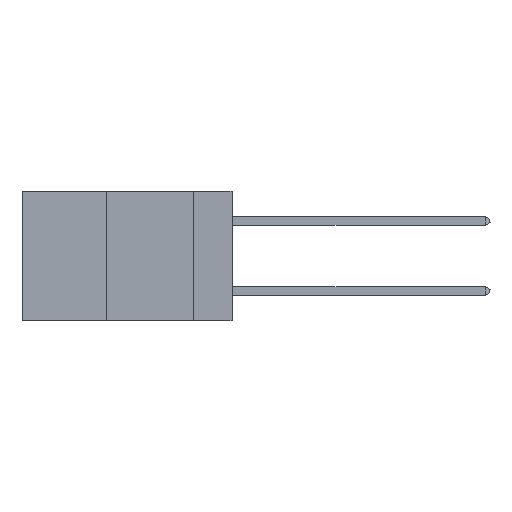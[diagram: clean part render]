
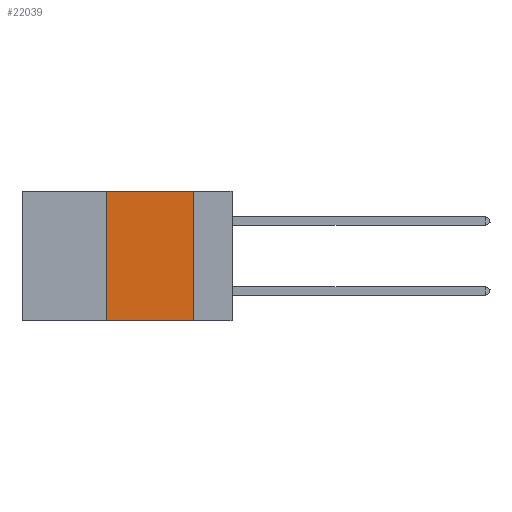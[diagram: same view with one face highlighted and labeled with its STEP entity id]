
A CAD part, left-side view. The second image highlights one B-rep face of the part: STEP entity #22039.
In plain terms, the highlighted planar face has unit normal (-1, 0, 0).
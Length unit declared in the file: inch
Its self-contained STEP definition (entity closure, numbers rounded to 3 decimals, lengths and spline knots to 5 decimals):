
#2424 = CARTESIAN_POINT ( 'NONE',  ( 0., 0.6, -0.37 ) ) ;
#3313 = DIRECTION ( 'NONE',  ( 0., 0., -1. ) ) ;
#3922 = VERTEX_POINT ( 'NONE', #30902 ) ;
#4229 = DIRECTION ( 'NONE',  ( 0., 0., -1. ) ) ;
#4431 = VECTOR ( 'NONE', #3313, 39.37008 ) ;
#4483 = ORIENTED_EDGE ( 'NONE', *, *, #11120, .F. ) ;
#6160 = VECTOR ( 'NONE', #17784, 39.37008 ) ;
#6839 = PLANE ( 'NONE',  #32558 ) ;
#6882 = VECTOR ( 'NONE', #17306, 39.37008 ) ;
#11120 = EDGE_CURVE ( 'NONE', #24749, #3922, #34038, .T. ) ;
#14887 = VECTOR ( 'NONE', #26249, 39.37008 ) ;
#14952 = CARTESIAN_POINT ( 'NONE',  ( 0., 0.6, 0. ) ) ;
#14987 = VERTEX_POINT ( 'NONE', #24565 ) ;
#15161 = CARTESIAN_POINT ( 'NONE',  ( 0., 0.6, 0. ) ) ;
#17306 = DIRECTION ( 'NONE',  ( 0., 0., 1. ) ) ;
#17784 = DIRECTION ( 'NONE',  ( 0., -1., 0. ) ) ;
#17951 = ORIENTED_EDGE ( 'NONE', *, *, #23624, .F. ) ;
#18876 = EDGE_LOOP ( 'NONE', ( #17951, #4483, #28363, #30797 ) ) ;
#19497 = EDGE_CURVE ( 'NONE', #29787, #14987, #21762, .T. ) ;
#20151 = DIRECTION ( 'NONE',  ( 1., 0., 0. ) ) ;
#21762 = LINE ( 'NONE', #2424, #14887 ) ;
#22039 = ADVANCED_FACE ( 'NONE', ( #32158 ), #6839, .F. ) ;
#23624 = EDGE_CURVE ( 'NONE', #3922, #14987, #34014, .T. ) ;
#23632 = CARTESIAN_POINT ( 'NONE',  ( 0., 0.36, 0. ) ) ;
#24507 = CARTESIAN_POINT ( 'NONE',  ( 0., 0.11, 0. ) ) ;
#24565 = CARTESIAN_POINT ( 'NONE',  ( 0., 0.11, -0.37 ) ) ;
#24749 = VERTEX_POINT ( 'NONE', #23632 ) ;
#24965 = CARTESIAN_POINT ( 'NONE',  ( 0., 0.36, 0. ) ) ;
#26249 = DIRECTION ( 'NONE',  ( 0., -1., 0. ) ) ;
#27833 = LINE ( 'NONE', #24965, #6882 ) ;
#28363 = ORIENTED_EDGE ( 'NONE', *, *, #29269, .F. ) ;
#29269 = EDGE_CURVE ( 'NONE', #29787, #24749, #27833, .T. ) ;
#29787 = VERTEX_POINT ( 'NONE', #31382 ) ;
#30797 = ORIENTED_EDGE ( 'NONE', *, *, #19497, .T. ) ;
#30902 = CARTESIAN_POINT ( 'NONE',  ( 0., 0.11, 0. ) ) ;
#31382 = CARTESIAN_POINT ( 'NONE',  ( 0., 0.36, -0.37 ) ) ;
#32158 = FACE_OUTER_BOUND ( 'NONE', #18876, .T. ) ;
#32558 = AXIS2_PLACEMENT_3D ( 'NONE', #14952, #20151, #4229 ) ;
#34014 = LINE ( 'NONE', #24507, #4431 ) ;
#34038 = LINE ( 'NONE', #15161, #6160 ) ;
